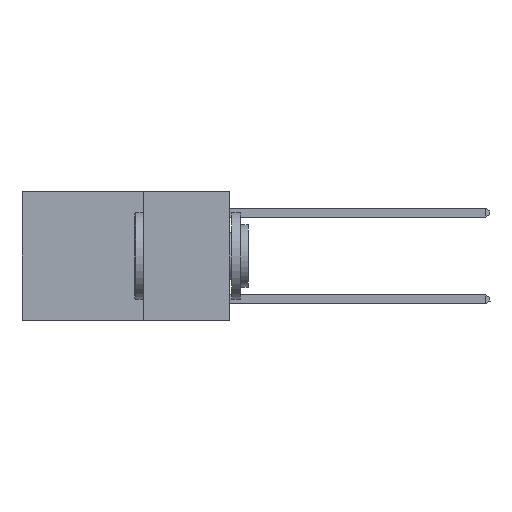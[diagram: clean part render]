
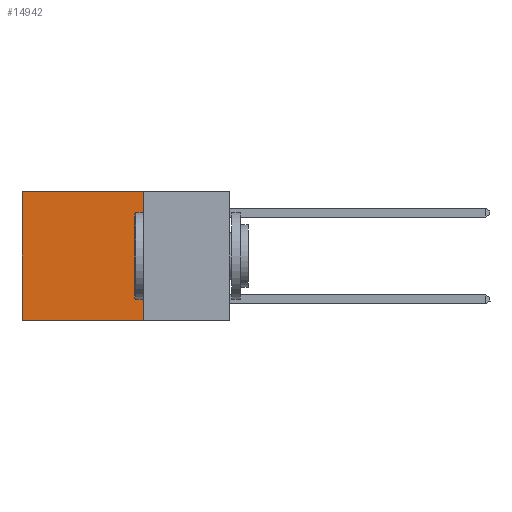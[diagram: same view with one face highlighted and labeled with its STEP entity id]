
A CAD part, left-side view. The second image highlights one B-rep face of the part: STEP entity #14942.
In plain terms, the highlighted planar face has unit normal (-1, 0, 0).
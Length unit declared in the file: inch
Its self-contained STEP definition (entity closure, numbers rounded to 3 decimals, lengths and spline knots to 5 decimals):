
#2186 = CARTESIAN_POINT ( 'NONE',  ( 0.2625, 0.25, 0. ) ) ;
#2371 = EDGE_LOOP ( 'NONE', ( #22183, #13588, #15518, #6675 ) ) ;
#2709 = EDGE_CURVE ( 'NONE', #9001, #13050, #4329, .T. ) ;
#2758 = CARTESIAN_POINT ( 'NONE',  ( 0.2625, 0.6, 0. ) ) ;
#2932 = VECTOR ( 'NONE', #12705, 39.37008 ) ;
#4329 = LINE ( 'NONE', #13278, #12823 ) ;
#4638 = DIRECTION ( 'NONE',  ( 1., 0., 0. ) ) ;
#4758 = LINE ( 'NONE', #9441, #13822 ) ;
#4913 = DIRECTION ( 'NONE',  ( 0., 0., -1. ) ) ;
#5435 = AXIS2_PLACEMENT_3D ( 'NONE', #17102, #4638, #18829 ) ;
#6675 = ORIENTED_EDGE ( 'NONE', *, *, #17447, .T. ) ;
#6679 = VERTEX_POINT ( 'NONE', #2186 ) ;
#7903 = VERTEX_POINT ( 'NONE', #15338 ) ;
#9001 = VERTEX_POINT ( 'NONE', #2758 ) ;
#9441 = CARTESIAN_POINT ( 'NONE',  ( 0.2625, 0.25, -0.37 ) ) ;
#9780 = PLANE ( 'NONE',  #5435 ) ;
#9862 = EDGE_CURVE ( 'NONE', #7903, #13050, #4758, .T. ) ;
#12093 = FACE_OUTER_BOUND ( 'NONE', #2371, .T. ) ;
#12705 = DIRECTION ( 'NONE',  ( 0., 1., 0. ) ) ;
#12823 = VECTOR ( 'NONE', #13354, 39.37008 ) ;
#13050 = VERTEX_POINT ( 'NONE', #16307 ) ;
#13278 = CARTESIAN_POINT ( 'NONE',  ( 0.2625, 0.6, 0. ) ) ;
#13354 = DIRECTION ( 'NONE',  ( 0., 0., -1. ) ) ;
#13588 = ORIENTED_EDGE ( 'NONE', *, *, #9862, .F. ) ;
#13822 = VECTOR ( 'NONE', #22070, 39.37008 ) ;
#14135 = EDGE_CURVE ( 'NONE', #6679, #7903, #17750, .T. ) ;
#14942 = ADVANCED_FACE ( 'NONE', ( #12093 ), #9780, .F. ) ;
#15338 = CARTESIAN_POINT ( 'NONE',  ( 0.2625, 0.25, -0.37 ) ) ;
#15518 = ORIENTED_EDGE ( 'NONE', *, *, #14135, .F. ) ;
#16307 = CARTESIAN_POINT ( 'NONE',  ( 0.2625, 0.6, -0.37 ) ) ;
#17102 = CARTESIAN_POINT ( 'NONE',  ( 0.2625, 0.25, 0. ) ) ;
#17447 = EDGE_CURVE ( 'NONE', #6679, #9001, #22436, .T. ) ;
#17750 = LINE ( 'NONE', #19425, #19705 ) ;
#17876 = CARTESIAN_POINT ( 'NONE',  ( 0.2625, 0.25, 0. ) ) ;
#18829 = DIRECTION ( 'NONE',  ( 0., 0., -1. ) ) ;
#19425 = CARTESIAN_POINT ( 'NONE',  ( 0.2625, 0.25, 0. ) ) ;
#19705 = VECTOR ( 'NONE', #4913, 39.37008 ) ;
#22070 = DIRECTION ( 'NONE',  ( 0., 1., 0. ) ) ;
#22183 = ORIENTED_EDGE ( 'NONE', *, *, #2709, .T. ) ;
#22436 = LINE ( 'NONE', #17876, #2932 ) ;
